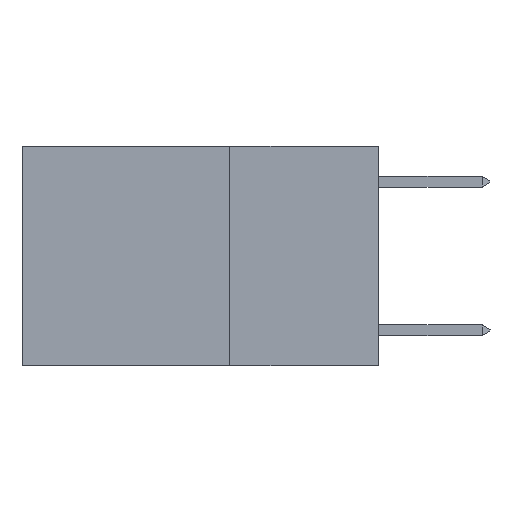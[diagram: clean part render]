
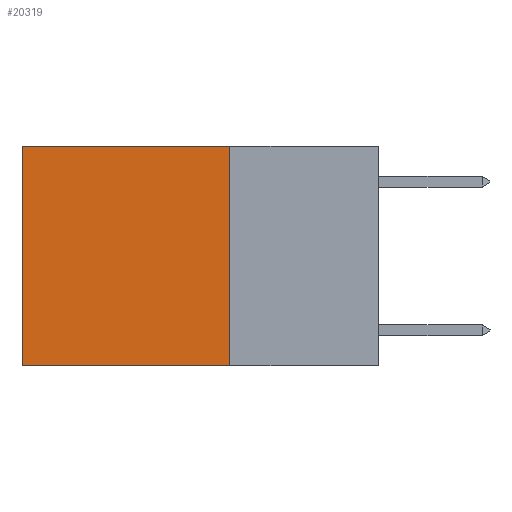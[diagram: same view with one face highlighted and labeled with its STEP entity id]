
A CAD part, left-side view. The second image highlights one B-rep face of the part: STEP entity #20319.
In plain terms, the highlighted planar face has unit normal (-1, 0, 0).
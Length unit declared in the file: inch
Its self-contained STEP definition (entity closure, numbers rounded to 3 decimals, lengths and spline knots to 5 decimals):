
#674 = CARTESIAN_POINT ( 'NONE',  ( 0.2625, 0.25, 0. ) ) ;
#1004 = DIRECTION ( 'NONE',  ( 0., 1., 0. ) ) ;
#2687 = CARTESIAN_POINT ( 'NONE',  ( 0.2625, 0.25, 0. ) ) ;
#3261 = AXIS2_PLACEMENT_3D ( 'NONE', #4305, #4167, #4122 ) ;
#3350 = EDGE_CURVE ( 'NONE', #9529, #11517, #7079, .T. ) ;
#3939 = VERTEX_POINT ( 'NONE', #15551 ) ;
#4122 = DIRECTION ( 'NONE',  ( 0., 0., -1. ) ) ;
#4167 = DIRECTION ( 'NONE',  ( 1., 0., 0. ) ) ;
#4305 = CARTESIAN_POINT ( 'NONE',  ( 0.2625, 0.25, 0. ) ) ;
#4308 = PLANE ( 'NONE',  #3261 ) ;
#4691 = VERTEX_POINT ( 'NONE', #14341 ) ;
#5783 = EDGE_CURVE ( 'NONE', #3939, #4691, #11039, .T. ) ;
#7079 = LINE ( 'NONE', #674, #7105 ) ;
#7105 = VECTOR ( 'NONE', #1004, 39.37008 ) ;
#7273 = CARTESIAN_POINT ( 'NONE',  ( 0.2625, 0.25, -0.37 ) ) ;
#7585 = ORIENTED_EDGE ( 'NONE', *, *, #3350, .T. ) ;
#8159 = DIRECTION ( 'NONE',  ( 0., 0., -1. ) ) ;
#8226 = CARTESIAN_POINT ( 'NONE',  ( 0.2625, 0.25, 0. ) ) ;
#8558 = ORIENTED_EDGE ( 'NONE', *, *, #10889, .T. ) ;
#9529 = VERTEX_POINT ( 'NONE', #2687 ) ;
#9969 = FACE_OUTER_BOUND ( 'NONE', #19320, .T. ) ;
#10845 = VECTOR ( 'NONE', #20179, 39.37008 ) ;
#10865 = ORIENTED_EDGE ( 'NONE', *, *, #19963, .F. ) ;
#10889 = EDGE_CURVE ( 'NONE', #11517, #4691, #18706, .T. ) ;
#11039 = LINE ( 'NONE', #7273, #10845 ) ;
#11517 = VERTEX_POINT ( 'NONE', #20351 ) ;
#12084 = VECTOR ( 'NONE', #8159, 39.37008 ) ;
#12286 = LINE ( 'NONE', #8226, #12084 ) ;
#13271 = DIRECTION ( 'NONE',  ( 0., 0., -1. ) ) ;
#14341 = CARTESIAN_POINT ( 'NONE',  ( 0.2625, 0.6, -0.37 ) ) ;
#15164 = CARTESIAN_POINT ( 'NONE',  ( 0.2625, 0.6, 0. ) ) ;
#15551 = CARTESIAN_POINT ( 'NONE',  ( 0.2625, 0.25, -0.37 ) ) ;
#16252 = ORIENTED_EDGE ( 'NONE', *, *, #5783, .F. ) ;
#18617 = VECTOR ( 'NONE', #13271, 39.37008 ) ;
#18706 = LINE ( 'NONE', #15164, #18617 ) ;
#19320 = EDGE_LOOP ( 'NONE', ( #8558, #16252, #10865, #7585 ) ) ;
#19963 = EDGE_CURVE ( 'NONE', #9529, #3939, #12286, .T. ) ;
#20179 = DIRECTION ( 'NONE',  ( 0., 1., 0. ) ) ;
#20319 = ADVANCED_FACE ( 'NONE', ( #9969 ), #4308, .F. ) ;
#20351 = CARTESIAN_POINT ( 'NONE',  ( 0.2625, 0.6, 0. ) ) ;
